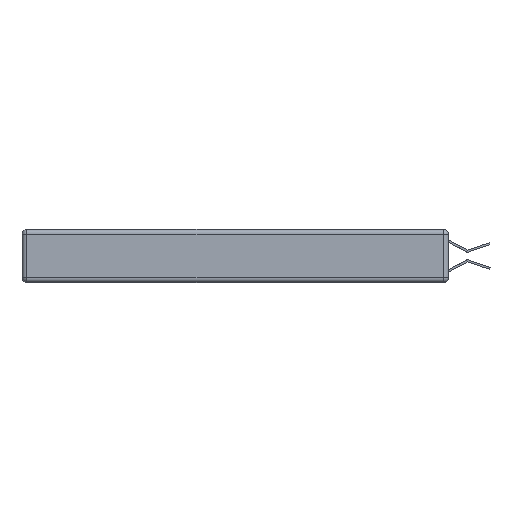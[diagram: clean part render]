
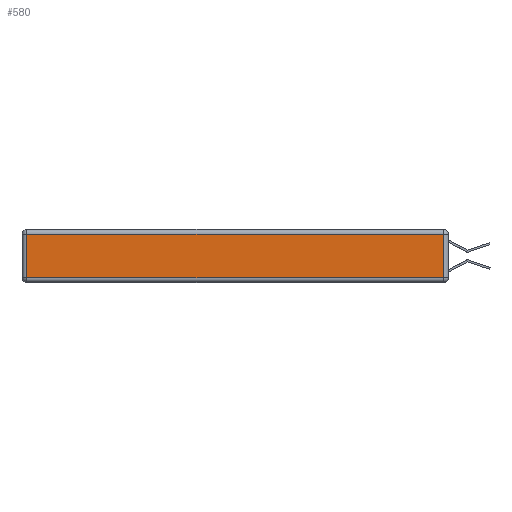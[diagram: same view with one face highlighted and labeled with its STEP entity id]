
A CAD part, left-side view. The second image highlights one B-rep face of the part: STEP entity #580.
In plain terms, the highlighted planar face has unit normal (-1, 0, 0).
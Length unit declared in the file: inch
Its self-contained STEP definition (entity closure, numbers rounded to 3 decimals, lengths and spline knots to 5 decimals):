
#348 = CARTESIAN_POINT ( 'NONE',  ( 0., 0.03, -0.313 ) ) ;
#552 = CARTESIAN_POINT ( 'NONE',  ( 0., 0., -0.313 ) ) ;
#580 = ADVANCED_FACE ( 'NONE', ( #4490 ), #7872, .T. ) ;
#694 = CARTESIAN_POINT ( 'NONE',  ( 0., 2.75, -0.03 ) ) ;
#944 = EDGE_CURVE ( 'NONE', #3892, #12697, #7432, .T. ) ;
#1187 = ORIENTED_EDGE ( 'NONE', *, *, #9973, .T. ) ;
#1453 = DIRECTION ( 'NONE',  ( 0., 0., 1. ) ) ;
#1773 = LINE ( 'NONE', #552, #12830 ) ;
#2384 = EDGE_CURVE ( 'NONE', #3816, #3892, #2423, .T. ) ;
#2423 = LINE ( 'NONE', #8552, #6388 ) ;
#3816 = VERTEX_POINT ( 'NONE', #348 ) ;
#3892 = VERTEX_POINT ( 'NONE', #6396 ) ;
#4490 = FACE_OUTER_BOUND ( 'NONE', #6019, .T. ) ;
#4664 = CARTESIAN_POINT ( 'NONE',  ( 0., 0., -0.343 ) ) ;
#4954 = VECTOR ( 'NONE', #8110, 39.37008 ) ;
#5396 = VECTOR ( 'NONE', #9992, 39.37008 ) ;
#5539 = ORIENTED_EDGE ( 'NONE', *, *, #944, .T. ) ;
#6019 = EDGE_LOOP ( 'NONE', ( #10653, #12027, #5539, #1187 ) ) ;
#6388 = VECTOR ( 'NONE', #13619, 39.37008 ) ;
#6396 = CARTESIAN_POINT ( 'NONE',  ( 0., 0.03, -0.03 ) ) ;
#6681 = VERTEX_POINT ( 'NONE', #10765 ) ;
#7432 = LINE ( 'NONE', #694, #4954 ) ;
#7804 = CARTESIAN_POINT ( 'NONE',  ( 0., 2.72, -0.343 ) ) ;
#7872 = PLANE ( 'NONE',  #11751 ) ;
#8110 = DIRECTION ( 'NONE',  ( 0., 1., 0. ) ) ;
#8552 = CARTESIAN_POINT ( 'NONE',  ( 0., 0.03, -0.343 ) ) ;
#9973 = EDGE_CURVE ( 'NONE', #12697, #6681, #12974, .T. ) ;
#9992 = DIRECTION ( 'NONE',  ( 0., 0., -1. ) ) ;
#10653 = ORIENTED_EDGE ( 'NONE', *, *, #11899, .T. ) ;
#10765 = CARTESIAN_POINT ( 'NONE',  ( 0., 2.72, -0.313 ) ) ;
#11751 = AXIS2_PLACEMENT_3D ( 'NONE', #4664, #12183, #1453 ) ;
#11781 = CARTESIAN_POINT ( 'NONE',  ( 0., 2.72, -0.03 ) ) ;
#11899 = EDGE_CURVE ( 'NONE', #6681, #3816, #1773, .T. ) ;
#12027 = ORIENTED_EDGE ( 'NONE', *, *, #2384, .T. ) ;
#12183 = DIRECTION ( 'NONE',  ( -1., 0., 0. ) ) ;
#12194 = DIRECTION ( 'NONE',  ( 0., -1., 0. ) ) ;
#12697 = VERTEX_POINT ( 'NONE', #11781 ) ;
#12830 = VECTOR ( 'NONE', #12194, 39.37008 ) ;
#12974 = LINE ( 'NONE', #7804, #5396 ) ;
#13619 = DIRECTION ( 'NONE',  ( 0., 0., 1. ) ) ;
